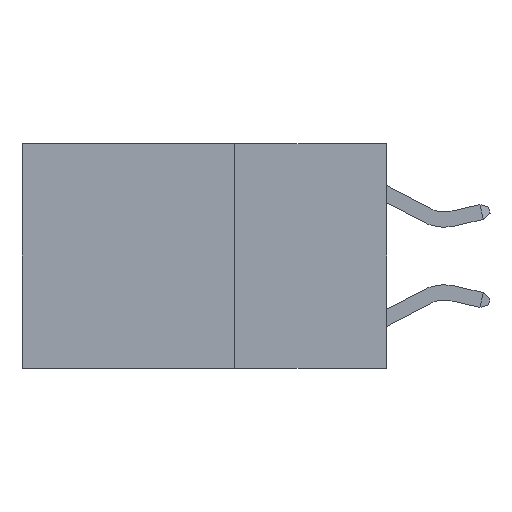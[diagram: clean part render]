
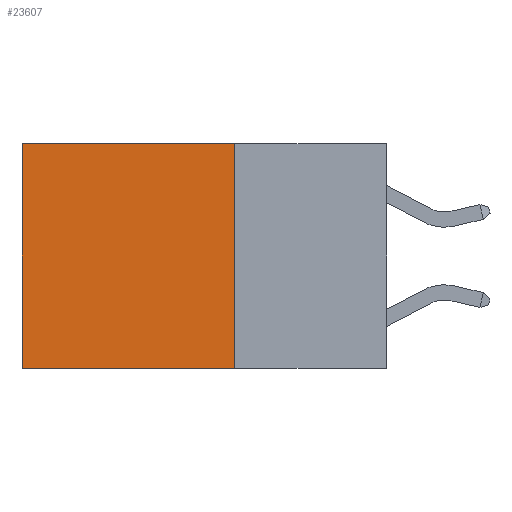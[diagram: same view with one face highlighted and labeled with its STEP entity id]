
A CAD part, left-side view. The second image highlights one B-rep face of the part: STEP entity #23607.
In plain terms, the highlighted planar face has unit normal (-1, 0, 0).
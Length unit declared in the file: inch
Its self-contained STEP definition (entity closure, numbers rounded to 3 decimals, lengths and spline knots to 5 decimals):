
#6 = ORIENTED_EDGE ( 'NONE', *, *, #4712, .T. ) ;
#89 = ORIENTED_EDGE ( 'NONE', *, *, #1060, .F. ) ;
#465 = CARTESIAN_POINT ( 'NONE',  ( 0.2625, 0.25, 0. ) ) ;
#1060 = EDGE_CURVE ( 'NONE', #4003, #5934, #2747, .T. ) ;
#2622 = DIRECTION ( 'NONE',  ( 0., 0., -1. ) ) ;
#2723 = ORIENTED_EDGE ( 'NONE', *, *, #9513, .F. ) ;
#2747 = LINE ( 'NONE', #24362, #23462 ) ;
#3422 = ORIENTED_EDGE ( 'NONE', *, *, #23102, .T. ) ;
#4003 = VERTEX_POINT ( 'NONE', #10083 ) ;
#4712 = EDGE_CURVE ( 'NONE', #4003, #25990, #18050, .T. ) ;
#5830 = CARTESIAN_POINT ( 'NONE',  ( 0.2625, 0.25, -0.37 ) ) ;
#5934 = VERTEX_POINT ( 'NONE', #5830 ) ;
#8110 = VECTOR ( 'NONE', #9463, 39.37008 ) ;
#9463 = DIRECTION ( 'NONE',  ( 0., 1., 0. ) ) ;
#9513 = EDGE_CURVE ( 'NONE', #5934, #11006, #13823, .T. ) ;
#10083 = CARTESIAN_POINT ( 'NONE',  ( 0.2625, 0.25, 0. ) ) ;
#10576 = CARTESIAN_POINT ( 'NONE',  ( 0.2625, 0.25, 0. ) ) ;
#11006 = VERTEX_POINT ( 'NONE', #18545 ) ;
#13002 = CARTESIAN_POINT ( 'NONE',  ( 0.2625, 0.6, 0. ) ) ;
#13687 = CARTESIAN_POINT ( 'NONE',  ( 0.2625, 0.25, -0.37 ) ) ;
#13768 = DIRECTION ( 'NONE',  ( 0., 0., -1. ) ) ;
#13823 = LINE ( 'NONE', #13687, #8110 ) ;
#13939 = DIRECTION ( 'NONE',  ( 0., 0., -1. ) ) ;
#14534 = VECTOR ( 'NONE', #13939, 39.37008 ) ;
#14985 = EDGE_LOOP ( 'NONE', ( #3422, #2723, #89, #6 ) ) ;
#15517 = DIRECTION ( 'NONE',  ( 1., 0., 0. ) ) ;
#16795 = AXIS2_PLACEMENT_3D ( 'NONE', #465, #15517, #2622 ) ;
#18050 = LINE ( 'NONE', #10576, #23032 ) ;
#18545 = CARTESIAN_POINT ( 'NONE',  ( 0.2625, 0.6, -0.37 ) ) ;
#19158 = DIRECTION ( 'NONE',  ( 0., 1., 0. ) ) ;
#19663 = PLANE ( 'NONE',  #16795 ) ;
#23032 = VECTOR ( 'NONE', #19158, 39.37008 ) ;
#23102 = EDGE_CURVE ( 'NONE', #25990, #11006, #25815, .T. ) ;
#23462 = VECTOR ( 'NONE', #13768, 39.37008 ) ;
#23607 = ADVANCED_FACE ( 'NONE', ( #24447 ), #19663, .F. ) ;
#24362 = CARTESIAN_POINT ( 'NONE',  ( 0.2625, 0.25, 0. ) ) ;
#24447 = FACE_OUTER_BOUND ( 'NONE', #14985, .T. ) ;
#25815 = LINE ( 'NONE', #26551, #14534 ) ;
#25990 = VERTEX_POINT ( 'NONE', #13002 ) ;
#26551 = CARTESIAN_POINT ( 'NONE',  ( 0.2625, 0.6, 0. ) ) ;
